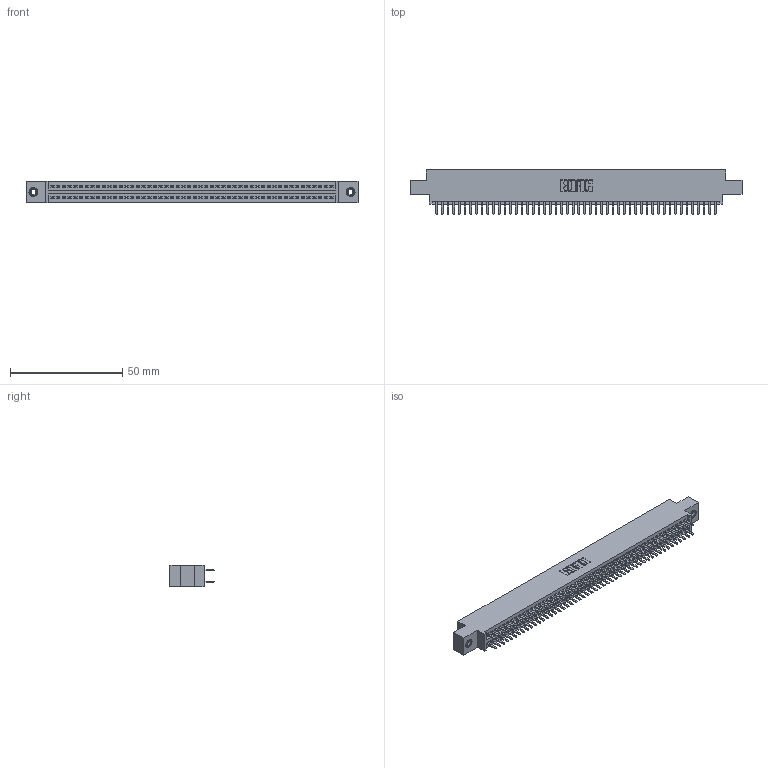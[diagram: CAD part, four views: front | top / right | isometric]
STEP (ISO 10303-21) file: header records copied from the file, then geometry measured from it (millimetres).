
FILE_DESCRIPTION (( 'STEP AP203' ), '1' );
FILE_NAME ('345-100-520-808.STEP', '2019-11-02T14:20:12', ( '' ), ( '' ), 'SwSTEP 2.0', 'SolidWorks 2016', '' );
FILE_SCHEMA (( 'CONFIG_CONTROL_DESIGN' ));
Length unit declared in the file: inch
Products named in the file (4): 345-100-520-808; 345-250-001_345-250-003-102; 345-292-001_345-293-120; 345 Part_0.170 Offset - 0.156 Dia-TI
Assembly tree (103 placements, depth 2):
  345-100-520-808
    345 Part_0.170 Offset - 0.156 Dia-TI
    345-292-001_345-293-120  x100
    345-250-001_345-250-003-102  x2
Bounding box: 148.21 x 19.68 x 9.4 mm (x, y, z)
Volume: 14307.6 mm3; surface area: 21367.3 mm2
Topology: 103 solids, 103 shells, 5590 faces, 16189 edges, 10518 vertices
Faces by surface type: plane 3616, cylinder 1958, cone 12, torus 4
Entity records: 39586 total; most frequent: CARTESIAN_POINT 6623, ORIENTED_EDGE 6538, DIRECTION 5843, EDGE_CURVE 3269, LINE 2913, VECTOR 2913, VERTEX_POINT 2172, AXIS2_PLACEMENT_3D 1465
